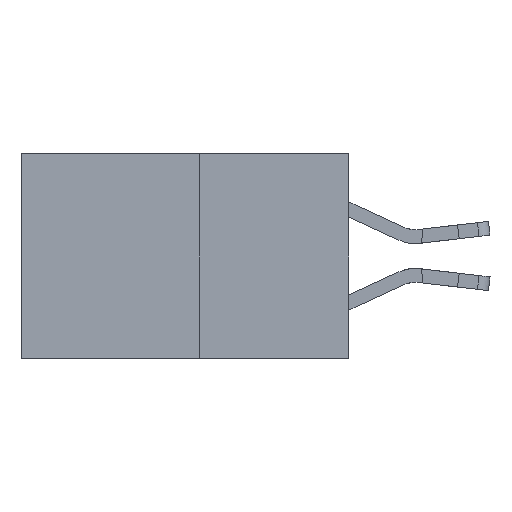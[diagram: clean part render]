
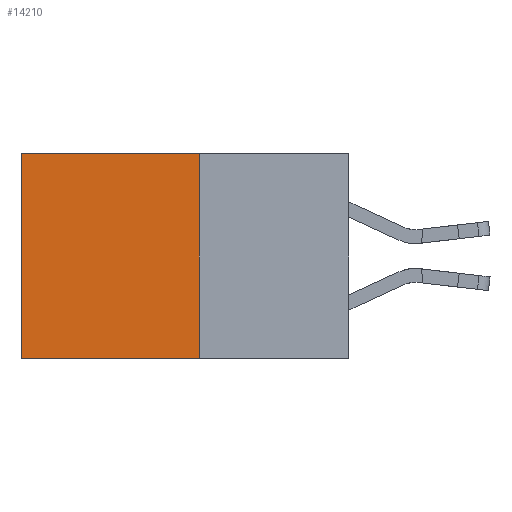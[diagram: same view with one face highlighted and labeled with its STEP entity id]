
A CAD part, left-side view. The second image highlights one B-rep face of the part: STEP entity #14210.
In plain terms, the highlighted planar face has unit normal (-1, 0, 0).
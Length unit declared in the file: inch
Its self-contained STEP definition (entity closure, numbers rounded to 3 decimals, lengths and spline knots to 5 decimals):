
#859 = EDGE_LOOP ( 'NONE', ( #11868, #8877, #18966, #2385 ) ) ;
#1899 = DIRECTION ( 'NONE',  ( 0., 1., 0. ) ) ;
#2033 = LINE ( 'NONE', #7052, #10721 ) ;
#2385 = ORIENTED_EDGE ( 'NONE', *, *, #4218, .T. ) ;
#3200 = CARTESIAN_POINT ( 'NONE',  ( 0.277, 0.59, 0. ) ) ;
#3466 = VERTEX_POINT ( 'NONE', #3864 ) ;
#3749 = LINE ( 'NONE', #11070, #15232 ) ;
#3864 = CARTESIAN_POINT ( 'NONE',  ( 0.277, 0.27, -0.37 ) ) ;
#4218 = EDGE_CURVE ( 'NONE', #17241, #6776, #13166, .T. ) ;
#4327 = VERTEX_POINT ( 'NONE', #14875 ) ;
#6151 = EDGE_CURVE ( 'NONE', #3466, #4327, #10339, .T. ) ;
#6776 = VERTEX_POINT ( 'NONE', #3200 ) ;
#7052 = CARTESIAN_POINT ( 'NONE',  ( 0.277, 0.27, -0.37 ) ) ;
#8859 = VECTOR ( 'NONE', #15420, 39.37008 ) ;
#8877 = ORIENTED_EDGE ( 'NONE', *, *, #6151, .F. ) ;
#9651 = CARTESIAN_POINT ( 'NONE',  ( 0.277, 0.27, -0.37 ) ) ;
#10034 = CARTESIAN_POINT ( 'NONE',  ( 0.277, 0.27, -0.37 ) ) ;
#10339 = LINE ( 'NONE', #10034, #15661 ) ;
#10721 = VECTOR ( 'NONE', #13527, 39.37008 ) ;
#11070 = CARTESIAN_POINT ( 'NONE',  ( 0.277, 0.59, -0.37 ) ) ;
#11282 = DIRECTION ( 'NONE',  ( 0., 0., -1. ) ) ;
#11868 = ORIENTED_EDGE ( 'NONE', *, *, #14143, .T. ) ;
#12608 = EDGE_CURVE ( 'NONE', #17241, #3466, #2033, .T. ) ;
#13166 = LINE ( 'NONE', #15494, #8859 ) ;
#13527 = DIRECTION ( 'NONE',  ( 0., 0., -1. ) ) ;
#14143 = EDGE_CURVE ( 'NONE', #6776, #4327, #3749, .T. ) ;
#14210 = ADVANCED_FACE ( 'NONE', ( #18018 ), #16123, .F. ) ;
#14875 = CARTESIAN_POINT ( 'NONE',  ( 0.277, 0.59, -0.37 ) ) ;
#15232 = VECTOR ( 'NONE', #15983, 39.37008 ) ;
#15253 = CARTESIAN_POINT ( 'NONE',  ( 0.277, 0.27, 0. ) ) ;
#15420 = DIRECTION ( 'NONE',  ( 0., 1., 0. ) ) ;
#15494 = CARTESIAN_POINT ( 'NONE',  ( 0.277, 0.27, 0. ) ) ;
#15661 = VECTOR ( 'NONE', #1899, 39.37008 ) ;
#15983 = DIRECTION ( 'NONE',  ( 0., 0., -1. ) ) ;
#16030 = AXIS2_PLACEMENT_3D ( 'NONE', #9651, #21025, #11282 ) ;
#16123 = PLANE ( 'NONE',  #16030 ) ;
#17241 = VERTEX_POINT ( 'NONE', #15253 ) ;
#18018 = FACE_OUTER_BOUND ( 'NONE', #859, .T. ) ;
#18966 = ORIENTED_EDGE ( 'NONE', *, *, #12608, .F. ) ;
#21025 = DIRECTION ( 'NONE',  ( 1., 0., 0. ) ) ;
